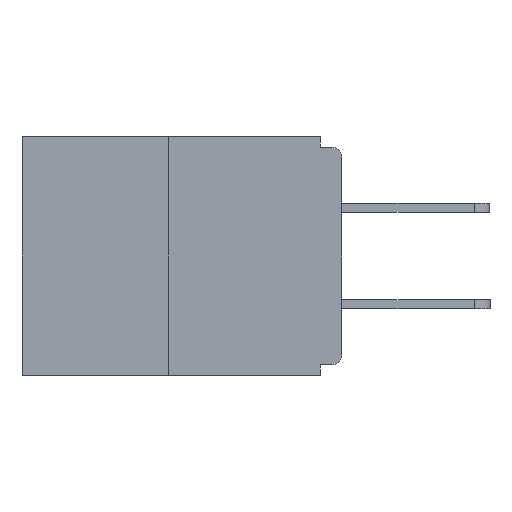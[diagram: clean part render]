
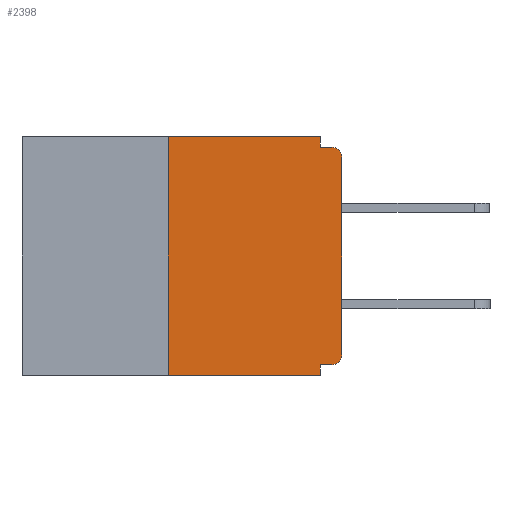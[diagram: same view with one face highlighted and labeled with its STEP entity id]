
A CAD part, left-side view. The second image highlights one B-rep face of the part: STEP entity #2398.
In plain terms, the highlighted planar face has unit normal (-1, 0, 0).
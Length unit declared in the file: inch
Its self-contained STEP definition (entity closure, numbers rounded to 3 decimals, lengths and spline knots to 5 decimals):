
#253 = AXIS2_PLACEMENT_3D ( 'NONE', #6340, #408, #3397 ) ;
#408 = DIRECTION ( 'NONE',  ( -1., 0., 0. ) ) ;
#642 = CIRCLE ( 'NONE', #12579, 0.015 ) ;
#819 = CARTESIAN_POINT ( 'NONE',  ( 0., 0.031, 0. ) ) ;
#1021 = LINE ( 'NONE', #1062, #7404 ) ;
#1042 = LINE ( 'NONE', #5733, #3551 ) ;
#1062 = CARTESIAN_POINT ( 'NONE',  ( 0., 0.46, -0.343 ) ) ;
#1203 = VERTEX_POINT ( 'NONE', #13547 ) ;
#1454 = EDGE_LOOP ( 'NONE', ( #18398, #4861, #13298, #6522, #1468, #2295, #12631, #18272, #8420, #9148 ) ) ;
#1468 = ORIENTED_EDGE ( 'NONE', *, *, #7063, .F. ) ;
#1847 = EDGE_CURVE ( 'NONE', #4783, #18169, #6994, .T. ) ;
#2033 = CIRCLE ( 'NONE', #253, 0.015 ) ;
#2295 = ORIENTED_EDGE ( 'NONE', *, *, #7157, .T. ) ;
#2398 = ADVANCED_FACE ( 'NONE', ( #10387 ), #10722, .F. ) ;
#2535 = VECTOR ( 'NONE', #4798, 39.37008 ) ;
#2571 = DIRECTION ( 'NONE',  ( 0., 0., -1. ) ) ;
#3120 = EDGE_CURVE ( 'NONE', #13881, #7660, #1021, .T. ) ;
#3168 = CARTESIAN_POINT ( 'NONE',  ( 0., 0.46, 0. ) ) ;
#3397 = DIRECTION ( 'NONE',  ( 0., 0., -1. ) ) ;
#3551 = VECTOR ( 'NONE', #6034, 39.37008 ) ;
#3755 = LINE ( 'NONE', #6098, #18795 ) ;
#4130 = VERTEX_POINT ( 'NONE', #11781 ) ;
#4276 = VECTOR ( 'NONE', #2571, 39.37008 ) ;
#4433 = VERTEX_POINT ( 'NONE', #13229 ) ;
#4542 = DIRECTION ( 'NONE',  ( 0., -1., 0. ) ) ;
#4783 = VERTEX_POINT ( 'NONE', #819 ) ;
#4798 = DIRECTION ( 'NONE',  ( 0., 0., -1. ) ) ;
#4861 = ORIENTED_EDGE ( 'NONE', *, *, #8785, .F. ) ;
#4917 = CARTESIAN_POINT ( 'NONE',  ( 0., 0.25, 0. ) ) ;
#4918 = CARTESIAN_POINT ( 'NONE',  ( 0., 0.031, -0.343 ) ) ;
#4952 = DIRECTION ( 'NONE',  ( 0., -1., 0. ) ) ;
#5733 = CARTESIAN_POINT ( 'NONE',  ( 0., 0.25, 0. ) ) ;
#6034 = DIRECTION ( 'NONE',  ( 0., 0., 1. ) ) ;
#6098 = CARTESIAN_POINT ( 'NONE',  ( 0., 0.46, 0. ) ) ;
#6340 = CARTESIAN_POINT ( 'NONE',  ( 0., 0.015, -0.313 ) ) ;
#6522 = ORIENTED_EDGE ( 'NONE', *, *, #11760, .F. ) ;
#6994 = LINE ( 'NONE', #18425, #4276 ) ;
#7063 = EDGE_CURVE ( 'NONE', #4130, #9246, #15682, .T. ) ;
#7157 = EDGE_CURVE ( 'NONE', #4130, #12617, #2033, .T. ) ;
#7290 = CARTESIAN_POINT ( 'NONE',  ( 0., 0., -0.313 ) ) ;
#7404 = VECTOR ( 'NONE', #4542, 39.37008 ) ;
#7660 = VERTEX_POINT ( 'NONE', #4918 ) ;
#7762 = EDGE_CURVE ( 'NONE', #4433, #1203, #642, .T. ) ;
#7983 = VECTOR ( 'NONE', #11754, 39.37008 ) ;
#8420 = ORIENTED_EDGE ( 'NONE', *, *, #18076, .F. ) ;
#8785 = EDGE_CURVE ( 'NONE', #13881, #10492, #1042, .T. ) ;
#8876 = EDGE_CURVE ( 'NONE', #10492, #4783, #3755, .T. ) ;
#8909 = CARTESIAN_POINT ( 'NONE',  ( 0., 0.031, -0.328 ) ) ;
#9148 = ORIENTED_EDGE ( 'NONE', *, *, #1847, .F. ) ;
#9246 = VERTEX_POINT ( 'NONE', #8909 ) ;
#10307 = AXIS2_PLACEMENT_3D ( 'NONE', #3168, #13361, #15146 ) ;
#10387 = FACE_OUTER_BOUND ( 'NONE', #1454, .T. ) ;
#10473 = CARTESIAN_POINT ( 'NONE',  ( 0., 0., 0. ) ) ;
#10492 = VERTEX_POINT ( 'NONE', #4917 ) ;
#10500 = CARTESIAN_POINT ( 'NONE',  ( 0., 0.031, -0.343 ) ) ;
#10722 = PLANE ( 'NONE',  #10307 ) ;
#11116 = DIRECTION ( 'NONE',  ( 0., 0., -1. ) ) ;
#11754 = DIRECTION ( 'NONE',  ( 0., 1., 0. ) ) ;
#11760 = EDGE_CURVE ( 'NONE', #9246, #7660, #18709, .T. ) ;
#11781 = CARTESIAN_POINT ( 'NONE',  ( 0., 0.015, -0.328 ) ) ;
#12554 = LINE ( 'NONE', #13204, #13669 ) ;
#12579 = AXIS2_PLACEMENT_3D ( 'NONE', #13971, #13859, #11116 ) ;
#12617 = VERTEX_POINT ( 'NONE', #7290 ) ;
#12631 = ORIENTED_EDGE ( 'NONE', *, *, #14380, .T. ) ;
#13003 = VECTOR ( 'NONE', #17464, 39.37008 ) ;
#13204 = CARTESIAN_POINT ( 'NONE',  ( 0., 0., -0.015 ) ) ;
#13229 = CARTESIAN_POINT ( 'NONE',  ( 0., 0., -0.03 ) ) ;
#13298 = ORIENTED_EDGE ( 'NONE', *, *, #3120, .T. ) ;
#13361 = DIRECTION ( 'NONE',  ( 1., 0., 0. ) ) ;
#13454 = CARTESIAN_POINT ( 'NONE',  ( 0., 0., -0.328 ) ) ;
#13547 = CARTESIAN_POINT ( 'NONE',  ( 0., 0.015, -0.015 ) ) ;
#13669 = VECTOR ( 'NONE', #16104, 39.37008 ) ;
#13859 = DIRECTION ( 'NONE',  ( -1., 0., 0. ) ) ;
#13881 = VERTEX_POINT ( 'NONE', #17176 ) ;
#13971 = CARTESIAN_POINT ( 'NONE',  ( 0., 0.015, -0.03 ) ) ;
#14365 = LINE ( 'NONE', #10473, #13003 ) ;
#14380 = EDGE_CURVE ( 'NONE', #12617, #4433, #14365, .T. ) ;
#15146 = DIRECTION ( 'NONE',  ( 0., 0., -1. ) ) ;
#15682 = LINE ( 'NONE', #13454, #7983 ) ;
#16104 = DIRECTION ( 'NONE',  ( 0., -1., 0. ) ) ;
#17176 = CARTESIAN_POINT ( 'NONE',  ( 0., 0.25, -0.343 ) ) ;
#17464 = DIRECTION ( 'NONE',  ( 0., 0., 1. ) ) ;
#17828 = CARTESIAN_POINT ( 'NONE',  ( 0., 0.031, -0.015 ) ) ;
#18076 = EDGE_CURVE ( 'NONE', #18169, #1203, #12554, .T. ) ;
#18169 = VERTEX_POINT ( 'NONE', #17828 ) ;
#18272 = ORIENTED_EDGE ( 'NONE', *, *, #7762, .T. ) ;
#18398 = ORIENTED_EDGE ( 'NONE', *, *, #8876, .F. ) ;
#18425 = CARTESIAN_POINT ( 'NONE',  ( 0., 0.031, 0. ) ) ;
#18709 = LINE ( 'NONE', #10500, #2535 ) ;
#18795 = VECTOR ( 'NONE', #4952, 39.37008 ) ;
